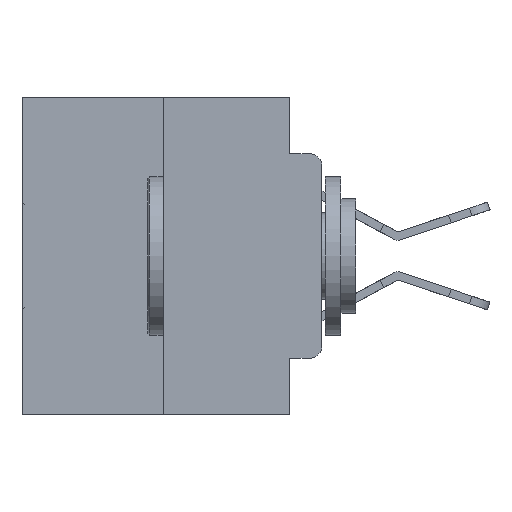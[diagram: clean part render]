
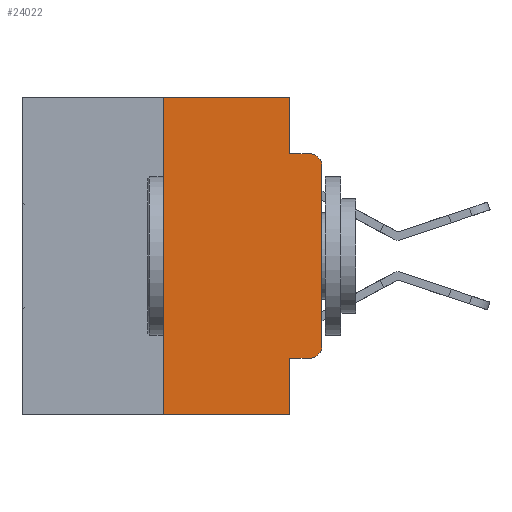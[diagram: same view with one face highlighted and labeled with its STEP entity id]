
A CAD part, left-side view. The second image highlights one B-rep face of the part: STEP entity #24022.
In plain terms, the highlighted planar face has unit normal (-1, 0, 0).
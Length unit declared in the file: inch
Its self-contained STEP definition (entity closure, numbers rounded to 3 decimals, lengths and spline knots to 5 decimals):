
#104 = CARTESIAN_POINT ( 'NONE',  ( 0., 0.25, 0. ) ) ;
#1062 = DIRECTION ( 'NONE',  ( 0., -1., 0. ) ) ;
#1147 = VERTEX_POINT ( 'NONE', #28375 ) ;
#1446 = VERTEX_POINT ( 'NONE', #13365 ) ;
#1581 = VERTEX_POINT ( 'NONE', #4086 ) ;
#2902 = CARTESIAN_POINT ( 'NONE',  ( 0., 0.051, -0.4115 ) ) ;
#3085 = CARTESIAN_POINT ( 'NONE',  ( 0., 0.051, -0.5 ) ) ;
#3284 = DIRECTION ( 'NONE',  ( -1., 0., 0. ) ) ;
#3308 = DIRECTION ( 'NONE',  ( 1., 0., 0. ) ) ;
#3567 = FACE_OUTER_BOUND ( 'NONE', #7318, .T. ) ;
#3995 = ORIENTED_EDGE ( 'NONE', *, *, #5657, .T. ) ;
#4086 = CARTESIAN_POINT ( 'NONE',  ( 0., 0., -0.3915 ) ) ;
#4105 = CARTESIAN_POINT ( 'NONE',  ( 0., 0., -0.1085 ) ) ;
#4533 = LINE ( 'NONE', #17634, #12238 ) ;
#4715 = VECTOR ( 'NONE', #28091, 39.37008 ) ;
#4731 = VECTOR ( 'NONE', #28546, 39.37008 ) ;
#5041 = VERTEX_POINT ( 'NONE', #26178 ) ;
#5580 = ORIENTED_EDGE ( 'NONE', *, *, #20093, .F. ) ;
#5637 = ORIENTED_EDGE ( 'NONE', *, *, #10763, .T. ) ;
#5657 = EDGE_CURVE ( 'NONE', #1581, #8886, #15990, .T. ) ;
#5697 = ORIENTED_EDGE ( 'NONE', *, *, #13885, .T. ) ;
#7056 = ORIENTED_EDGE ( 'NONE', *, *, #14522, .F. ) ;
#7318 = EDGE_LOOP ( 'NONE', ( #3995, #17977, #7056, #13894, #20968, #5580, #5637, #27825, #17767, #5697 ) ) ;
#8393 = EDGE_CURVE ( 'NONE', #31221, #5041, #30217, .T. ) ;
#8886 = VERTEX_POINT ( 'NONE', #4105 ) ;
#8928 = CARTESIAN_POINT ( 'NONE',  ( 0., 0.051, 0. ) ) ;
#9245 = DIRECTION ( 'NONE',  ( 0., -1., 0. ) ) ;
#9711 = CARTESIAN_POINT ( 'NONE',  ( 0., 0.051, -0.0885 ) ) ;
#9884 = CARTESIAN_POINT ( 'NONE',  ( 0., 0.25, 0. ) ) ;
#10763 = EDGE_CURVE ( 'NONE', #1147, #12025, #19970, .T. ) ;
#11480 = VERTEX_POINT ( 'NONE', #25373 ) ;
#11691 = AXIS2_PLACEMENT_3D ( 'NONE', #15583, #22858, #18293 ) ;
#11929 = VECTOR ( 'NONE', #24471, 39.37008 ) ;
#12025 = VERTEX_POINT ( 'NONE', #3085 ) ;
#12238 = VECTOR ( 'NONE', #27583, 39.37008 ) ;
#12826 = EDGE_CURVE ( 'NONE', #5041, #26980, #24851, .T. ) ;
#13020 = DIRECTION ( 'NONE',  ( 0., 0., 1. ) ) ;
#13365 = CARTESIAN_POINT ( 'NONE',  ( 0., 0.02, -0.4115 ) ) ;
#13414 = VERTEX_POINT ( 'NONE', #16057 ) ;
#13885 = EDGE_CURVE ( 'NONE', #1446, #1581, #25945, .T. ) ;
#13894 = ORIENTED_EDGE ( 'NONE', *, *, #12826, .F. ) ;
#14522 = EDGE_CURVE ( 'NONE', #26980, #13414, #20485, .T. ) ;
#15385 = DIRECTION ( 'NONE',  ( 0., -1., 0. ) ) ;
#15583 = CARTESIAN_POINT ( 'NONE',  ( 0., 0.02, -0.3915 ) ) ;
#15672 = CARTESIAN_POINT ( 'NONE',  ( 0., 0.02, -0.1085 ) ) ;
#15990 = LINE ( 'NONE', #22887, #23781 ) ;
#15994 = EDGE_CURVE ( 'NONE', #11480, #1446, #16521, .T. ) ;
#16057 = CARTESIAN_POINT ( 'NONE',  ( 0., 0.02, -0.0885 ) ) ;
#16521 = LINE ( 'NONE', #2902, #25449 ) ;
#16591 = EDGE_CURVE ( 'NONE', #11480, #12025, #4533, .T. ) ;
#17634 = CARTESIAN_POINT ( 'NONE',  ( 0., 0.051, 0. ) ) ;
#17767 = ORIENTED_EDGE ( 'NONE', *, *, #15994, .T. ) ;
#17977 = ORIENTED_EDGE ( 'NONE', *, *, #21268, .T. ) ;
#18062 = DIRECTION ( 'NONE',  ( 0., 0., -1. ) ) ;
#18293 = DIRECTION ( 'NONE',  ( 0., 0., -1. ) ) ;
#19970 = LINE ( 'NONE', #26693, #30809 ) ;
#20093 = EDGE_CURVE ( 'NONE', #1147, #31221, #27142, .T. ) ;
#20485 = LINE ( 'NONE', #22210, #11929 ) ;
#20590 = DIRECTION ( 'NONE',  ( 0., 0., -1. ) ) ;
#20934 = VECTOR ( 'NONE', #1062, 39.37008 ) ;
#20968 = ORIENTED_EDGE ( 'NONE', *, *, #8393, .F. ) ;
#21268 = EDGE_CURVE ( 'NONE', #8886, #13414, #22864, .T. ) ;
#22210 = CARTESIAN_POINT ( 'NONE',  ( 0., 0.051, -0.0885 ) ) ;
#22858 = DIRECTION ( 'NONE',  ( -1., 0., 0. ) ) ;
#22864 = CIRCLE ( 'NONE', #23636, 0.02 ) ;
#22887 = CARTESIAN_POINT ( 'NONE',  ( 0., 0., 0. ) ) ;
#23636 = AXIS2_PLACEMENT_3D ( 'NONE', #15672, #3284, #18062 ) ;
#23781 = VECTOR ( 'NONE', #13020, 39.37008 ) ;
#24022 = ADVANCED_FACE ( 'NONE', ( #3567 ), #28143, .F. ) ;
#24471 = DIRECTION ( 'NONE',  ( 0., -1., 0. ) ) ;
#24851 = LINE ( 'NONE', #8928, #4731 ) ;
#25373 = CARTESIAN_POINT ( 'NONE',  ( 0., 0.051, -0.4115 ) ) ;
#25449 = VECTOR ( 'NONE', #15385, 39.37008 ) ;
#25768 = AXIS2_PLACEMENT_3D ( 'NONE', #27930, #3308, #20590 ) ;
#25945 = CIRCLE ( 'NONE', #11691, 0.02 ) ;
#26178 = CARTESIAN_POINT ( 'NONE',  ( 0., 0.051, 0. ) ) ;
#26693 = CARTESIAN_POINT ( 'NONE',  ( 0., 0.473, -0.5 ) ) ;
#26980 = VERTEX_POINT ( 'NONE', #9711 ) ;
#27142 = LINE ( 'NONE', #104, #4715 ) ;
#27583 = DIRECTION ( 'NONE',  ( 0., 0., -1. ) ) ;
#27825 = ORIENTED_EDGE ( 'NONE', *, *, #16591, .F. ) ;
#27930 = CARTESIAN_POINT ( 'NONE',  ( 0., 0.473, 0. ) ) ;
#28091 = DIRECTION ( 'NONE',  ( 0., 0., 1. ) ) ;
#28143 = PLANE ( 'NONE',  #25768 ) ;
#28375 = CARTESIAN_POINT ( 'NONE',  ( 0., 0.25, -0.5 ) ) ;
#28546 = DIRECTION ( 'NONE',  ( 0., 0., -1. ) ) ;
#30217 = LINE ( 'NONE', #32006, #20934 ) ;
#30809 = VECTOR ( 'NONE', #9245, 39.37008 ) ;
#31221 = VERTEX_POINT ( 'NONE', #9884 ) ;
#32006 = CARTESIAN_POINT ( 'NONE',  ( 0., 0.473, 0. ) ) ;
